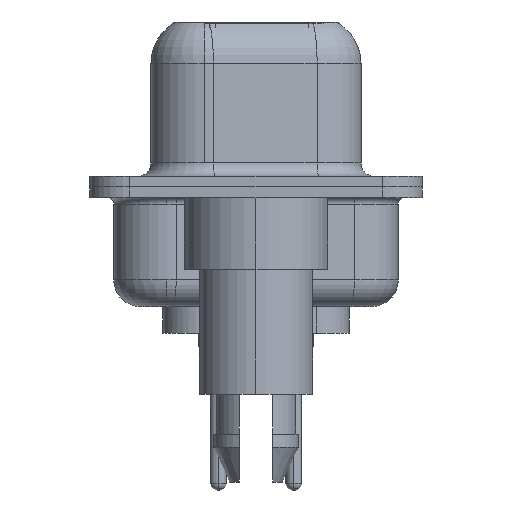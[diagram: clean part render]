
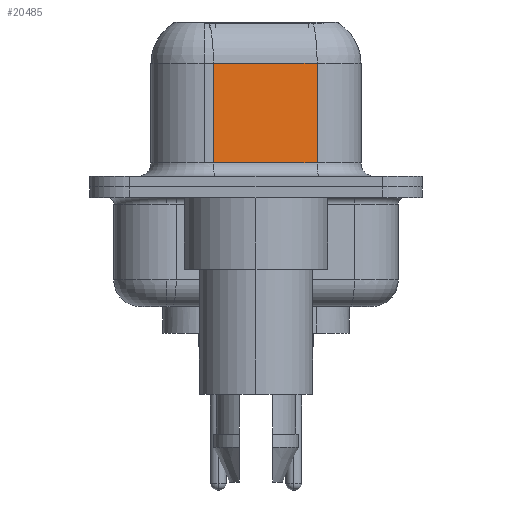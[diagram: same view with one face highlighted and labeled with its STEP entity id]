
A CAD part, left-side view. The second image highlights one B-rep face of the part: STEP entity #20485.
In plain terms, the highlighted planar face has unit normal (-0.985, -0.174, 0).
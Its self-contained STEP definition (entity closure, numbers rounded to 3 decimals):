
#324 = EDGE_CURVE ( 'NONE', #12084, #11880, #14684, .T. ) ;
#693 = CARTESIAN_POINT ( 'NONE',  ( 5.043, -2.297, 6.4 ) ) ;
#2529 = DIRECTION ( 'NONE',  ( 0., 0., -1. ) ) ;
#2673 = CARTESIAN_POINT ( 'NONE',  ( 4.355, 1.603, 6.4 ) ) ;
#4140 = LINE ( 'NONE', #693, #20792 ) ;
#4192 = CARTESIAN_POINT ( 'NONE',  ( 5.043, -2.297, 4.65 ) ) ;
#4572 = ORIENTED_EDGE ( 'NONE', *, *, #7358, .T. ) ;
#7012 = CARTESIAN_POINT ( 'NONE',  ( 5.043, -2.297, 6.4 ) ) ;
#7312 = ORIENTED_EDGE ( 'NONE', *, *, #18867, .F. ) ;
#7358 = EDGE_CURVE ( 'NONE', #11880, #13467, #14554, .T. ) ;
#7625 = AXIS2_PLACEMENT_3D ( 'NONE', #7012, #15770, #16452 ) ;
#7661 = DIRECTION ( 'NONE',  ( 0., 0., -1. ) ) ;
#8741 = FACE_OUTER_BOUND ( 'NONE', #22121, .T. ) ;
#8887 = DIRECTION ( 'NONE',  ( 0.174, -0.985, 0. ) ) ;
#9321 = CARTESIAN_POINT ( 'NONE',  ( 5.043, -2.297, 0.9 ) ) ;
#9955 = CARTESIAN_POINT ( 'NONE',  ( 4.355, 1.603, 4.65 ) ) ;
#10630 = VECTOR ( 'NONE', #8887, 1000. ) ;
#11013 = DIRECTION ( 'NONE',  ( -0.174, 0.985, 0. ) ) ;
#11617 = CARTESIAN_POINT ( 'NONE',  ( 5.043, -2.297, 4.65 ) ) ;
#11770 = ORIENTED_EDGE ( 'NONE', *, *, #324, .T. ) ;
#11880 = VERTEX_POINT ( 'NONE', #9955 ) ;
#12084 = VERTEX_POINT ( 'NONE', #11617 ) ;
#13467 = VERTEX_POINT ( 'NONE', #19428 ) ;
#14554 = LINE ( 'NONE', #2673, #18545 ) ;
#14684 = LINE ( 'NONE', #4192, #21033 ) ;
#15309 = VERTEX_POINT ( 'NONE', #9321 ) ;
#15555 = ORIENTED_EDGE ( 'NONE', *, *, #17333, .T. ) ;
#15770 = DIRECTION ( 'NONE',  ( 0.985, 0.174, 0. ) ) ;
#15922 = CARTESIAN_POINT ( 'NONE',  ( 5.043, -2.297, 0.9 ) ) ;
#16452 = DIRECTION ( 'NONE',  ( -0.174, 0.985, 0. ) ) ;
#16963 = LINE ( 'NONE', #15922, #10630 ) ;
#17333 = EDGE_CURVE ( 'NONE', #13467, #15309, #16963, .T. ) ;
#18545 = VECTOR ( 'NONE', #7661, 1000. ) ;
#18867 = EDGE_CURVE ( 'NONE', #12084, #15309, #4140, .T. ) ;
#19428 = CARTESIAN_POINT ( 'NONE',  ( 4.355, 1.603, 0.9 ) ) ;
#20485 = ADVANCED_FACE ( 'NONE', ( #8741 ), #21037, .F. ) ;
#20792 = VECTOR ( 'NONE', #2529, 1000. ) ;
#21033 = VECTOR ( 'NONE', #11013, 1000. ) ;
#21037 = PLANE ( 'NONE',  #7625 ) ;
#22121 = EDGE_LOOP ( 'NONE', ( #7312, #11770, #4572, #15555 ) ) ;
